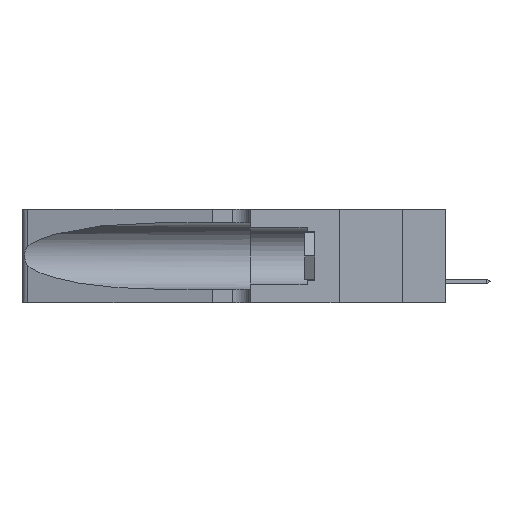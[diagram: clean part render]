
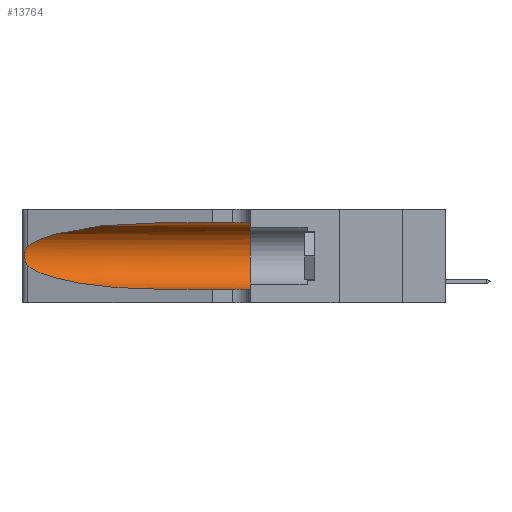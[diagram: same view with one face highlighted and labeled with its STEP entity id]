
A CAD part, left-side view. The second image highlights one B-rep face of the part: STEP entity #13764.
In plain terms, the highlighted cylindrical face has radius 3.308 mm (diameter 6.617 mm), a partial arc.
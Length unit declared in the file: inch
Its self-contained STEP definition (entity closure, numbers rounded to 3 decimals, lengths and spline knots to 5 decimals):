
#2810 = AXIS2_PLACEMENT_3D ( 'NONE', #19546, #44230, #37454 ) ;
#3128 = CARTESIAN_POINT ( 'NONE',  ( 0.18966, 0.96281, 0.31525 ) ) ;
#3604 = CARTESIAN_POINT ( 'NONE',  ( 0.25854, 1.2359, 0.20912 ) ) ;
#3744 = CARTESIAN_POINT ( 'NONE',  ( 0.25787, 1.23484, 0.2124 ) ) ;
#4467 = EDGE_LOOP ( 'NONE', ( #18683, #40287, #10900, #12209, #34764, #26909 ) ) ;
#5417 = CARTESIAN_POINT ( 'NONE',  ( 0.25487, 1.22718, 0.14631 ) ) ;
#5673 = VERTEX_POINT ( 'NONE', #12304 ) ;
#6105 = CARTESIAN_POINT ( 'NONE',  ( 0.1305, 0.72297, 0.31525 ) ) ;
#6362 = CARTESIAN_POINT ( 'NONE',  ( 0.1305, 0.72297, 0.05475 ) ) ;
#6711 = CARTESIAN_POINT ( 'NONE',  ( 0.25487, 1.22718, 0.22369 ) ) ;
#6738 = CARTESIAN_POINT ( 'NONE',  ( 0.25639, 1.23184, 0.21858 ) ) ;
#6825 = AXIS2_PLACEMENT_3D ( 'NONE', #36100, #7536, #18787 ) ;
#6849 = EDGE_CURVE ( 'NONE', #8923, #35597, #42418, .T. ) ;
#7043 = LINE ( 'NONE', #17391, #10362 ) ;
#7338 = CARTESIAN_POINT ( 'NONE',  ( 0.26075, 1.23896, 0.178 ) ) ;
#7441 =( BOUNDED_CURVE ( )  B_SPLINE_CURVE ( 3, ( #6105, #3128, #34398, #6711 ),
 .UNSPECIFIED., .F., .F. ) 
 B_SPLINE_CURVE_WITH_KNOTS ( ( 4, 4 ),
 ( 1.5708, 2.84003 ),
 .UNSPECIFIED. ) 
 CURVE ( )  GEOMETRIC_REPRESENTATION_ITEM ( )  RATIONAL_B_SPLINE_CURVE ( ( 1., 0.87, 0.87, 1. ) ) 
 REPRESENTATION_ITEM ( '' )  );
#7536 = DIRECTION ( 'NONE',  ( 0., -1., 0. ) ) ;
#7605 = EDGE_CURVE ( 'NONE', #8923, #17818, #7441, .T. ) ;
#8724 = CYLINDRICAL_SURFACE ( 'NONE', #6825, 0.13025 ) ;
#8923 = VERTEX_POINT ( 'NONE', #12246 ) ;
#9466 = CARTESIAN_POINT ( 'NONE',  ( 0.1305, 1.61858, 0.31525 ) ) ;
#10362 = VECTOR ( 'NONE', #35445, 39.37008 ) ;
#10900 = ORIENTED_EDGE ( 'NONE', *, *, #29548, .T. ) ;
#12209 = ORIENTED_EDGE ( 'NONE', *, *, #38476, .T. ) ;
#12246 = CARTESIAN_POINT ( 'NONE',  ( 0.1305, 0.72297, 0.31525 ) ) ;
#12304 = CARTESIAN_POINT ( 'NONE',  ( 0.1305, 0.35, 0.05475 ) ) ;
#13764 = ADVANCED_FACE ( 'NONE', ( #16484 ), #8724, .F. ) ;
#14401 = CARTESIAN_POINT ( 'NONE',  ( 0.25555, 1.22993, 0.14849 ) ) ;
#16484 = FACE_OUTER_BOUND ( 'NONE', #4467, .T. ) ;
#16704 = DIRECTION ( 'NONE',  ( 0., -1., 0. ) ) ;
#17391 = CARTESIAN_POINT ( 'NONE',  ( 0.1305, 1.61858, 0.05475 ) ) ;
#17818 = VERTEX_POINT ( 'NONE', #43775 ) ;
#18683 = ORIENTED_EDGE ( 'NONE', *, *, #7605, .T. ) ;
#18787 = DIRECTION ( 'NONE',  ( 0., 0., -1. ) ) ;
#18850 = CIRCLE ( 'NONE', #2810, 0.13025 ) ;
#19403 = VERTEX_POINT ( 'NONE', #40438 ) ;
#19546 = CARTESIAN_POINT ( 'NONE',  ( 0.1305, 0.35, 0.185 ) ) ;
#21928 = CARTESIAN_POINT ( 'NONE',  ( 0.1305, 0.72297, 0.05475 ) ) ;
#22441 =( BOUNDED_CURVE ( )  B_SPLINE_CURVE ( 3, ( #5417, #27363, #44787, #6362 ),
 .UNSPECIFIED., .F., .F. ) 
 B_SPLINE_CURVE_WITH_KNOTS ( ( 4, 4 ),
 ( 3.44316, 4.71239 ),
 .UNSPECIFIED. ) 
 CURVE ( )  GEOMETRIC_REPRESENTATION_ITEM ( )  RATIONAL_B_SPLINE_CURVE ( ( 1., 0.87, 0.87, 1. ) ) 
 REPRESENTATION_ITEM ( '' )  );
#24485 = CARTESIAN_POINT ( 'NONE',  ( 0.26018, 1.23835, 0.19895 ) ) ;
#26909 = ORIENTED_EDGE ( 'NONE', *, *, #6849, .F. ) ;
#27363 = CARTESIAN_POINT ( 'NONE',  ( 0.2373, 1.15595, 0.08982 ) ) ;
#27539 = VECTOR ( 'NONE', #16704, 39.37008 ) ;
#28342 = CARTESIAN_POINT ( 'NONE',  ( 0.26017, 1.23833, 0.17102 ) ) ;
#28487 = CARTESIAN_POINT ( 'NONE',  ( 0.26075, 1.23896, 0.19203 ) ) ;
#29548 = EDGE_CURVE ( 'NONE', #19403, #33294, #22441, .T. ) ;
#31517 = B_SPLINE_CURVE_WITH_KNOTS ( 'NONE', 3,
 ( #35437, #42488, #6738, #3744, #3604, #24485, #28487, #7338, #28342, #32038, #45475, #38687, #14401, #41926 ),
 .UNSPECIFIED., .F., .F.,
 ( 4, 2, 2, 2, 2, 2, 4 ),
 ( 0., 0.00027, 0.00053, 0.00107, 0.0016, 0.00187, 0.00214 ),
 .UNSPECIFIED. ) ;
#32038 = CARTESIAN_POINT ( 'NONE',  ( 0.25856, 1.23593, 0.16098 ) ) ;
#33294 = VERTEX_POINT ( 'NONE', #21928 ) ;
#34398 = CARTESIAN_POINT ( 'NONE',  ( 0.2373, 1.15595, 0.28018 ) ) ;
#34764 = ORIENTED_EDGE ( 'NONE', *, *, #42376, .F. ) ;
#35433 = EDGE_CURVE ( 'NONE', #17818, #19403, #31517, .T. ) ;
#35437 = CARTESIAN_POINT ( 'NONE',  ( 0.25487, 1.22718, 0.22369 ) ) ;
#35445 = DIRECTION ( 'NONE',  ( 0., -1., 0. ) ) ;
#35597 = VERTEX_POINT ( 'NONE', #42786 ) ;
#36100 = CARTESIAN_POINT ( 'NONE',  ( 0.1305, 1.61858, 0.185 ) ) ;
#37454 = DIRECTION ( 'NONE',  ( 0., 0., 1. ) ) ;
#38476 = EDGE_CURVE ( 'NONE', #33294, #5673, #7043, .T. ) ;
#38687 = CARTESIAN_POINT ( 'NONE',  ( 0.25639, 1.23186, 0.15144 ) ) ;
#40287 = ORIENTED_EDGE ( 'NONE', *, *, #35433, .T. ) ;
#40438 = CARTESIAN_POINT ( 'NONE',  ( 0.25487, 1.22718, 0.14631 ) ) ;
#41926 = CARTESIAN_POINT ( 'NONE',  ( 0.25487, 1.22718, 0.14631 ) ) ;
#42376 = EDGE_CURVE ( 'NONE', #35597, #5673, #18850, .T. ) ;
#42418 = LINE ( 'NONE', #9466, #27539 ) ;
#42488 = CARTESIAN_POINT ( 'NONE',  ( 0.25555, 1.22994, 0.2215 ) ) ;
#42786 = CARTESIAN_POINT ( 'NONE',  ( 0.1305, 0.35, 0.31525 ) ) ;
#43775 = CARTESIAN_POINT ( 'NONE',  ( 0.25487, 1.22718, 0.22369 ) ) ;
#44230 = DIRECTION ( 'NONE',  ( 0., 1., 0. ) ) ;
#44787 = CARTESIAN_POINT ( 'NONE',  ( 0.18966, 0.96281, 0.05475 ) ) ;
#45475 = CARTESIAN_POINT ( 'NONE',  ( 0.25789, 1.23486, 0.15765 ) ) ;
